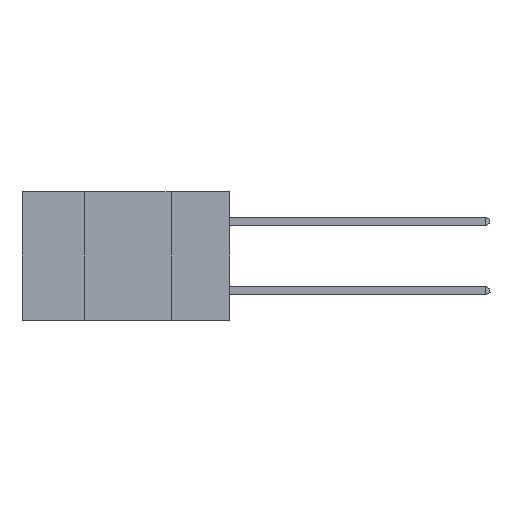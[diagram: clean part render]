
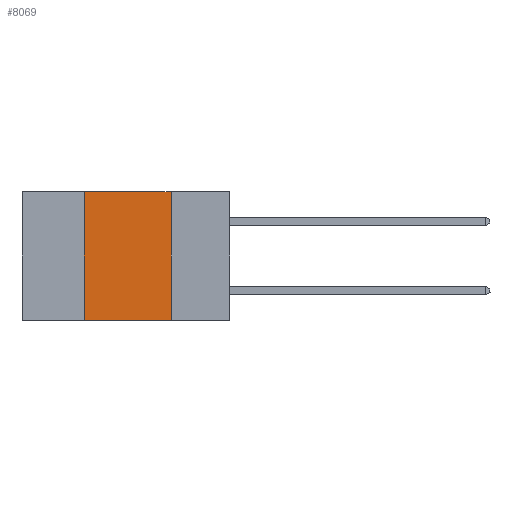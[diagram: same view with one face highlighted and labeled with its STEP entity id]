
A CAD part, left-side view. The second image highlights one B-rep face of the part: STEP entity #8069.
In plain terms, the highlighted planar face has unit normal (-1, 0, 0).
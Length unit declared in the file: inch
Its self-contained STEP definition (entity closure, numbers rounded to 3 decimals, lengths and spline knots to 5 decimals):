
#10 = CARTESIAN_POINT ( 'NONE',  ( 0., 0.42, -0.37 ) ) ;
#168 = VECTOR ( 'NONE', #4892, 39.37008 ) ;
#901 = FACE_OUTER_BOUND ( 'NONE', #13782, .T. ) ;
#2674 = CARTESIAN_POINT ( 'NONE',  ( 0., 0.17, -0.37 ) ) ;
#2872 = VECTOR ( 'NONE', #10410, 39.37008 ) ;
#3075 = CARTESIAN_POINT ( 'NONE',  ( 0., 0.6, 0. ) ) ;
#4892 = DIRECTION ( 'NONE',  ( 0., 0., 1. ) ) ;
#5067 = CARTESIAN_POINT ( 'NONE',  ( 0., 0.17, 0. ) ) ;
#5222 = VERTEX_POINT ( 'NONE', #2674 ) ;
#8069 = ADVANCED_FACE ( 'NONE', ( #901 ), #27214, .F. ) ;
#8338 = AXIS2_PLACEMENT_3D ( 'NONE', #3075, #29591, #15309 ) ;
#10410 = DIRECTION ( 'NONE',  ( 0., -1., 0. ) ) ;
#10795 = CARTESIAN_POINT ( 'NONE',  ( 0., 0.17, 0. ) ) ;
#11313 = EDGE_CURVE ( 'NONE', #25841, #5222, #16024, .T. ) ;
#12080 = ORIENTED_EDGE ( 'NONE', *, *, #26513, .F. ) ;
#12845 = CARTESIAN_POINT ( 'NONE',  ( 0., 0.6, 0. ) ) ;
#13337 = VECTOR ( 'NONE', #20416, 39.37008 ) ;
#13782 = EDGE_LOOP ( 'NONE', ( #23644, #12080, #15391, #25755 ) ) ;
#14679 = CARTESIAN_POINT ( 'NONE',  ( 0., 0.42, 0. ) ) ;
#15309 = DIRECTION ( 'NONE',  ( 0., 0., -1. ) ) ;
#15391 = ORIENTED_EDGE ( 'NONE', *, *, #17720, .F. ) ;
#16024 = LINE ( 'NONE', #30324, #27974 ) ;
#17720 = EDGE_CURVE ( 'NONE', #25841, #25819, #25967, .T. ) ;
#19699 = LINE ( 'NONE', #10795, #13337 ) ;
#20416 = DIRECTION ( 'NONE',  ( 0., 0., -1. ) ) ;
#20920 = EDGE_CURVE ( 'NONE', #21379, #5222, #19699, .T. ) ;
#21379 = VERTEX_POINT ( 'NONE', #5067 ) ;
#22163 = LINE ( 'NONE', #12845, #2872 ) ;
#23644 = ORIENTED_EDGE ( 'NONE', *, *, #20920, .F. ) ;
#25755 = ORIENTED_EDGE ( 'NONE', *, *, #11313, .T. ) ;
#25819 = VERTEX_POINT ( 'NONE', #28927 ) ;
#25841 = VERTEX_POINT ( 'NONE', #10 ) ;
#25967 = LINE ( 'NONE', #14679, #168 ) ;
#26513 = EDGE_CURVE ( 'NONE', #25819, #21379, #22163, .T. ) ;
#27214 = PLANE ( 'NONE',  #8338 ) ;
#27974 = VECTOR ( 'NONE', #30212, 39.37008 ) ;
#28927 = CARTESIAN_POINT ( 'NONE',  ( 0., 0.42, 0. ) ) ;
#29591 = DIRECTION ( 'NONE',  ( 1., 0., 0. ) ) ;
#30212 = DIRECTION ( 'NONE',  ( 0., -1., 0. ) ) ;
#30324 = CARTESIAN_POINT ( 'NONE',  ( 0., 0.6, -0.37 ) ) ;
